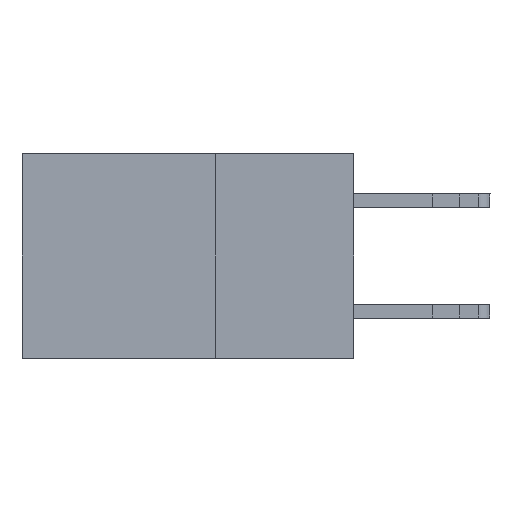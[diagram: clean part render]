
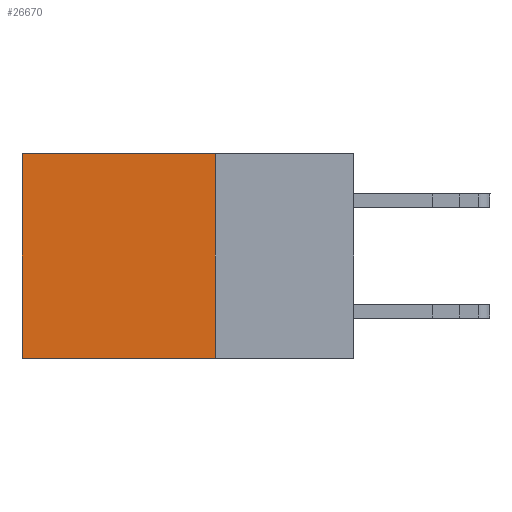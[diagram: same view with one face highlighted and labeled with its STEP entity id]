
A CAD part, left-side view. The second image highlights one B-rep face of the part: STEP entity #26670.
In plain terms, the highlighted planar face has unit normal (-1, 0, 0).
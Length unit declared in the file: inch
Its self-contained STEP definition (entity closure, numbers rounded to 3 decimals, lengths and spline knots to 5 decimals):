
#396 = LINE ( 'NONE', #35662, #35772 ) ;
#1775 = VERTEX_POINT ( 'NONE', #10141 ) ;
#4548 = CARTESIAN_POINT ( 'NONE',  ( 0.2875, 0.6, 0. ) ) ;
#5338 = LINE ( 'NONE', #10531, #20451 ) ;
#5625 = EDGE_CURVE ( 'NONE', #28561, #31917, #35126, .T. ) ;
#8854 = DIRECTION ( 'NONE',  ( 0., 0., -1. ) ) ;
#9208 = CARTESIAN_POINT ( 'NONE',  ( 0.2875, 0.25, 0. ) ) ;
#9392 = DIRECTION ( 'NONE',  ( 1., 0., 0. ) ) ;
#9682 = EDGE_CURVE ( 'NONE', #1775, #18964, #5338, .T. ) ;
#10141 = CARTESIAN_POINT ( 'NONE',  ( 0.2875, 0.25, 0. ) ) ;
#10293 = EDGE_LOOP ( 'NONE', ( #18456, #37364, #28387, #36481 ) ) ;
#10531 = CARTESIAN_POINT ( 'NONE',  ( 0.2875, 0.25, 0. ) ) ;
#10773 = EDGE_CURVE ( 'NONE', #18964, #31917, #396, .T. ) ;
#12832 = AXIS2_PLACEMENT_3D ( 'NONE', #9208, #9392, #21113 ) ;
#14297 = CARTESIAN_POINT ( 'NONE',  ( 0.2875, 0.6, -0.37 ) ) ;
#18456 = ORIENTED_EDGE ( 'NONE', *, *, #5625, .T. ) ;
#18591 = LINE ( 'NONE', #18779, #32778 ) ;
#18779 = CARTESIAN_POINT ( 'NONE',  ( 0.2875, 0.25, 0. ) ) ;
#18964 = VERTEX_POINT ( 'NONE', #33800 ) ;
#20311 = EDGE_CURVE ( 'NONE', #1775, #28561, #18591, .T. ) ;
#20451 = VECTOR ( 'NONE', #22226, 39.37008 ) ;
#21113 = DIRECTION ( 'NONE',  ( 0., 0., -1. ) ) ;
#22226 = DIRECTION ( 'NONE',  ( 0., 0., -1. ) ) ;
#23792 = DIRECTION ( 'NONE',  ( 0., 1., 0. ) ) ;
#24530 = CARTESIAN_POINT ( 'NONE',  ( 0.2875, 0.6, 0. ) ) ;
#24710 = DIRECTION ( 'NONE',  ( 0., 1., 0. ) ) ;
#26670 = ADVANCED_FACE ( 'NONE', ( #35478 ), #35665, .F. ) ;
#28387 = ORIENTED_EDGE ( 'NONE', *, *, #9682, .F. ) ;
#28561 = VERTEX_POINT ( 'NONE', #4548 ) ;
#31362 = VECTOR ( 'NONE', #8854, 39.37008 ) ;
#31917 = VERTEX_POINT ( 'NONE', #14297 ) ;
#32778 = VECTOR ( 'NONE', #24710, 39.37008 ) ;
#33800 = CARTESIAN_POINT ( 'NONE',  ( 0.2875, 0.25, -0.37 ) ) ;
#35126 = LINE ( 'NONE', #24530, #31362 ) ;
#35478 = FACE_OUTER_BOUND ( 'NONE', #10293, .T. ) ;
#35662 = CARTESIAN_POINT ( 'NONE',  ( 0.2875, 0.25, -0.37 ) ) ;
#35665 = PLANE ( 'NONE',  #12832 ) ;
#35772 = VECTOR ( 'NONE', #23792, 39.37008 ) ;
#36481 = ORIENTED_EDGE ( 'NONE', *, *, #20311, .T. ) ;
#37364 = ORIENTED_EDGE ( 'NONE', *, *, #10773, .F. ) ;
